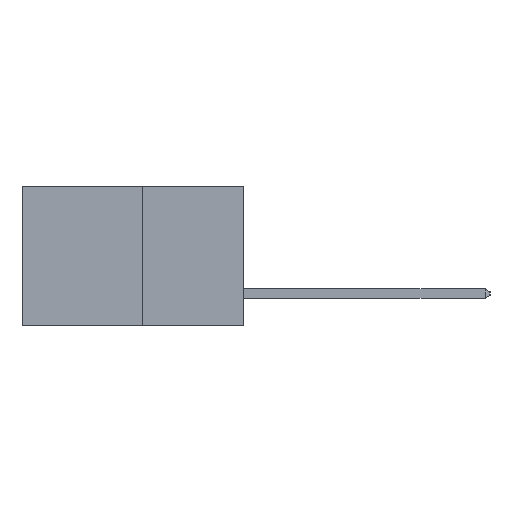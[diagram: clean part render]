
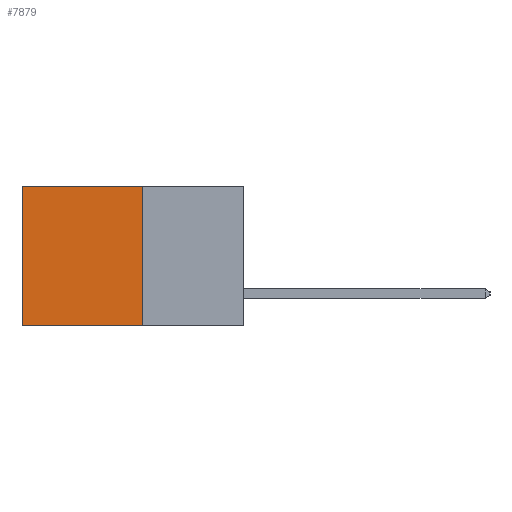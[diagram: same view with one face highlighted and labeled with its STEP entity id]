
A CAD part, left-side view. The second image highlights one B-rep face of the part: STEP entity #7879.
In plain terms, the highlighted planar face has unit normal (-1, 0, 0).
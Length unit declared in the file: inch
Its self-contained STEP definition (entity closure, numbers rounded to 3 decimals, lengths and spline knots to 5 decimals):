
#265 = CARTESIAN_POINT ( 'NONE',  ( 0.277, 0.27, -0.37 ) ) ;
#489 = VERTEX_POINT ( 'NONE', #265 ) ;
#756 = DIRECTION ( 'NONE',  ( 0., 0., -1. ) ) ;
#957 = ORIENTED_EDGE ( 'NONE', *, *, #12562, .F. ) ;
#1468 = DIRECTION ( 'NONE',  ( 0., 1., 0. ) ) ;
#2244 = DIRECTION ( 'NONE',  ( 0., 0., -1. ) ) ;
#2347 = LINE ( 'NONE', #21286, #20069 ) ;
#2516 = EDGE_CURVE ( 'NONE', #489, #19199, #11403, .T. ) ;
#3080 = DIRECTION ( 'NONE',  ( 0., 1., 0. ) ) ;
#6132 = VERTEX_POINT ( 'NONE', #7888 ) ;
#7324 = EDGE_CURVE ( 'NONE', #16056, #19199, #11831, .T. ) ;
#7879 = ADVANCED_FACE ( 'NONE', ( #21561 ), #9251, .F. ) ;
#7888 = CARTESIAN_POINT ( 'NONE',  ( 0.277, 0.27, 0. ) ) ;
#8695 = ORIENTED_EDGE ( 'NONE', *, *, #2516, .F. ) ;
#8750 = CARTESIAN_POINT ( 'NONE',  ( 0.277, 0.59, -0.37 ) ) ;
#9251 = PLANE ( 'NONE',  #14944 ) ;
#9288 = VECTOR ( 'NONE', #1468, 39.37008 ) ;
#10334 = EDGE_CURVE ( 'NONE', #6132, #16056, #13827, .T. ) ;
#10668 = CARTESIAN_POINT ( 'NONE',  ( 0.277, 0.59, 0. ) ) ;
#11016 = DIRECTION ( 'NONE',  ( 0., 0., -1. ) ) ;
#11403 = LINE ( 'NONE', #17774, #15354 ) ;
#11831 = LINE ( 'NONE', #17669, #19763 ) ;
#12562 = EDGE_CURVE ( 'NONE', #6132, #489, #2347, .T. ) ;
#13827 = LINE ( 'NONE', #21971, #9288 ) ;
#14944 = AXIS2_PLACEMENT_3D ( 'NONE', #16027, #21090, #11016 ) ;
#15354 = VECTOR ( 'NONE', #3080, 39.37008 ) ;
#16027 = CARTESIAN_POINT ( 'NONE',  ( 0.277, 0.27, -0.37 ) ) ;
#16056 = VERTEX_POINT ( 'NONE', #10668 ) ;
#16120 = ORIENTED_EDGE ( 'NONE', *, *, #7324, .T. ) ;
#17669 = CARTESIAN_POINT ( 'NONE',  ( 0.277, 0.59, -0.37 ) ) ;
#17774 = CARTESIAN_POINT ( 'NONE',  ( 0.277, 0.27, -0.37 ) ) ;
#17941 = ORIENTED_EDGE ( 'NONE', *, *, #10334, .T. ) ;
#19199 = VERTEX_POINT ( 'NONE', #8750 ) ;
#19763 = VECTOR ( 'NONE', #2244, 39.37008 ) ;
#20069 = VECTOR ( 'NONE', #756, 39.37008 ) ;
#21083 = EDGE_LOOP ( 'NONE', ( #16120, #8695, #957, #17941 ) ) ;
#21090 = DIRECTION ( 'NONE',  ( 1., 0., 0. ) ) ;
#21286 = CARTESIAN_POINT ( 'NONE',  ( 0.277, 0.27, -0.37 ) ) ;
#21561 = FACE_OUTER_BOUND ( 'NONE', #21083, .T. ) ;
#21971 = CARTESIAN_POINT ( 'NONE',  ( 0.277, 0.27, 0. ) ) ;
